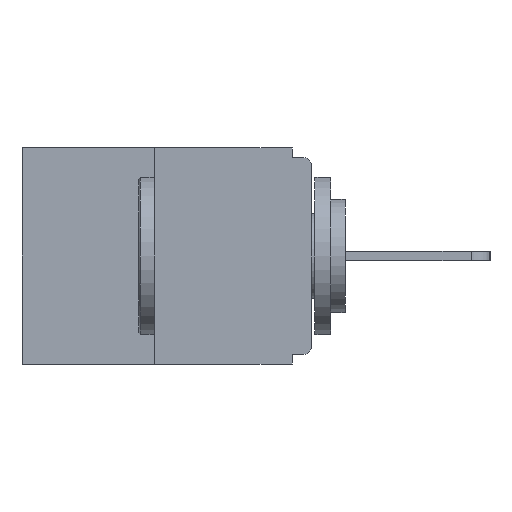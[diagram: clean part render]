
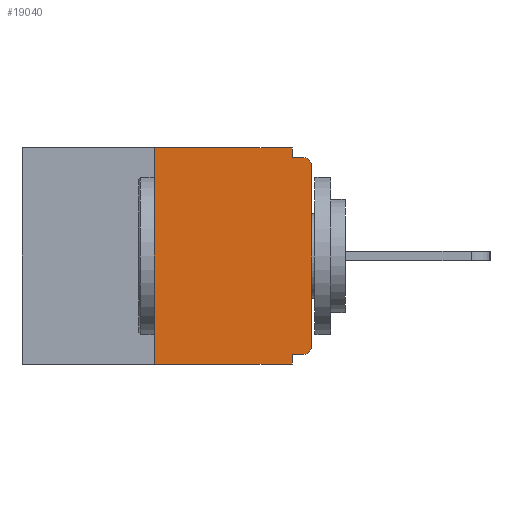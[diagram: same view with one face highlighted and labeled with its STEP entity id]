
A CAD part, left-side view. The second image highlights one B-rep face of the part: STEP entity #19040.
In plain terms, the highlighted planar face has unit normal (-1, 0, 0).
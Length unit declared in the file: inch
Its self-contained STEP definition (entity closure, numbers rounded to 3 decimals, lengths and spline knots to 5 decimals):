
#199 = VERTEX_POINT ( 'NONE', #11319 ) ;
#419 = LINE ( 'NONE', #11018, #18500 ) ;
#460 = DIRECTION ( 'NONE',  ( 1., 0., 0. ) ) ;
#535 = CARTESIAN_POINT ( 'NONE',  ( 0., 0.031, -0.343 ) ) ;
#539 = DIRECTION ( 'NONE',  ( 0., 0., -1. ) ) ;
#1986 = DIRECTION ( 'NONE',  ( 0., -1., 0. ) ) ;
#2222 = VERTEX_POINT ( 'NONE', #7398 ) ;
#2345 = CARTESIAN_POINT ( 'NONE',  ( 0., 0.46, 0. ) ) ;
#2422 = ORIENTED_EDGE ( 'NONE', *, *, #13037, .T. ) ;
#2543 = CARTESIAN_POINT ( 'NONE',  ( 0., 0., 0. ) ) ;
#2627 = VECTOR ( 'NONE', #21052, 39.37008 ) ;
#3037 = EDGE_CURVE ( 'NONE', #7523, #5427, #3733, .T. ) ;
#3152 = CARTESIAN_POINT ( 'NONE',  ( 0., 0.015, -0.03 ) ) ;
#3335 = CARTESIAN_POINT ( 'NONE',  ( 0., 0.031, -0.015 ) ) ;
#3733 = LINE ( 'NONE', #13937, #15692 ) ;
#4079 = EDGE_CURVE ( 'NONE', #18840, #16915, #9987, .T. ) ;
#4166 = ORIENTED_EDGE ( 'NONE', *, *, #6965, .F. ) ;
#4241 = DIRECTION ( 'NONE',  ( 0., -1., 0. ) ) ;
#4781 = CARTESIAN_POINT ( 'NONE',  ( 0., 0., -0.015 ) ) ;
#4887 = CARTESIAN_POINT ( 'NONE',  ( 0., 0.46, -0.343 ) ) ;
#4950 = DIRECTION ( 'NONE',  ( 0., 0., -1. ) ) ;
#5097 = DIRECTION ( 'NONE',  ( 0., 1., 0. ) ) ;
#5274 = CARTESIAN_POINT ( 'NONE',  ( 0., 0.25, 0. ) ) ;
#5427 = VERTEX_POINT ( 'NONE', #16603 ) ;
#5719 = EDGE_LOOP ( 'NONE', ( #16451, #10334, #20446, #6708, #17253, #20076, #2422, #19606, #4166, #11992 ) ) ;
#6475 = DIRECTION ( 'NONE',  ( 0., 0., 1. ) ) ;
#6708 = ORIENTED_EDGE ( 'NONE', *, *, #10070, .F. ) ;
#6965 = EDGE_CURVE ( 'NONE', #7738, #17714, #7440, .T. ) ;
#7297 = CIRCLE ( 'NONE', #14392, 0.015 ) ;
#7362 = EDGE_CURVE ( 'NONE', #199, #17811, #16793, .T. ) ;
#7398 = CARTESIAN_POINT ( 'NONE',  ( 0., 0., -0.03 ) ) ;
#7440 = LINE ( 'NONE', #4781, #19583 ) ;
#7523 = VERTEX_POINT ( 'NONE', #13383 ) ;
#7738 = VERTEX_POINT ( 'NONE', #3335 ) ;
#7961 = VECTOR ( 'NONE', #1986, 39.37008 ) ;
#8301 = EDGE_CURVE ( 'NONE', #18840, #199, #21797, .T. ) ;
#8455 = CARTESIAN_POINT ( 'NONE',  ( 0., 0., -0.313 ) ) ;
#8465 = CARTESIAN_POINT ( 'NONE',  ( 0., 0.015, -0.015 ) ) ;
#8633 = VECTOR ( 'NONE', #6475, 39.37008 ) ;
#8730 = DIRECTION ( 'NONE',  ( 0., -1., 0. ) ) ;
#8837 = EDGE_CURVE ( 'NONE', #7523, #14530, #7297, .T. ) ;
#9469 = VECTOR ( 'NONE', #8730, 39.37008 ) ;
#9909 = VECTOR ( 'NONE', #12599, 39.37008 ) ;
#9987 = LINE ( 'NONE', #4887, #9469 ) ;
#10070 = EDGE_CURVE ( 'NONE', #5427, #16915, #18637, .T. ) ;
#10184 = DIRECTION ( 'NONE',  ( 0., 0., -1. ) ) ;
#10214 = DIRECTION ( 'NONE',  ( -1., 0., 0. ) ) ;
#10334 = ORIENTED_EDGE ( 'NONE', *, *, #8301, .F. ) ;
#10362 = CARTESIAN_POINT ( 'NONE',  ( 0., 0.015, -0.313 ) ) ;
#10775 = CARTESIAN_POINT ( 'NONE',  ( 0., 0.031, 0. ) ) ;
#10934 = CARTESIAN_POINT ( 'NONE',  ( 0., 0.46, 0. ) ) ;
#11018 = CARTESIAN_POINT ( 'NONE',  ( 0., 0.031, 0. ) ) ;
#11319 = CARTESIAN_POINT ( 'NONE',  ( 0., 0.25, 0. ) ) ;
#11560 = CARTESIAN_POINT ( 'NONE',  ( 0., 0.031, -0.343 ) ) ;
#11992 = ORIENTED_EDGE ( 'NONE', *, *, #13576, .F. ) ;
#12591 = DIRECTION ( 'NONE',  ( 0., 0., -1. ) ) ;
#12599 = DIRECTION ( 'NONE',  ( 0., 0., -1. ) ) ;
#13037 = EDGE_CURVE ( 'NONE', #14530, #2222, #21090, .T. ) ;
#13159 = AXIS2_PLACEMENT_3D ( 'NONE', #10934, #460, #12591 ) ;
#13383 = CARTESIAN_POINT ( 'NONE',  ( 0., 0.015, -0.328 ) ) ;
#13576 = EDGE_CURVE ( 'NONE', #17811, #7738, #419, .T. ) ;
#13689 = CARTESIAN_POINT ( 'NONE',  ( 0., 0.25, -0.343 ) ) ;
#13937 = CARTESIAN_POINT ( 'NONE',  ( 0., 0., -0.328 ) ) ;
#14392 = AXIS2_PLACEMENT_3D ( 'NONE', #10362, #10214, #10184 ) ;
#14530 = VERTEX_POINT ( 'NONE', #8455 ) ;
#15085 = DIRECTION ( 'NONE',  ( -1., 0., 0. ) ) ;
#15692 = VECTOR ( 'NONE', #5097, 39.37008 ) ;
#16451 = ORIENTED_EDGE ( 'NONE', *, *, #7362, .F. ) ;
#16508 = EDGE_CURVE ( 'NONE', #2222, #17714, #20759, .T. ) ;
#16603 = CARTESIAN_POINT ( 'NONE',  ( 0., 0.031, -0.328 ) ) ;
#16793 = LINE ( 'NONE', #2345, #7961 ) ;
#16915 = VERTEX_POINT ( 'NONE', #11560 ) ;
#17253 = ORIENTED_EDGE ( 'NONE', *, *, #3037, .F. ) ;
#17714 = VERTEX_POINT ( 'NONE', #8465 ) ;
#17811 = VERTEX_POINT ( 'NONE', #10775 ) ;
#18500 = VECTOR ( 'NONE', #539, 39.37008 ) ;
#18637 = LINE ( 'NONE', #535, #9909 ) ;
#18840 = VERTEX_POINT ( 'NONE', #13689 ) ;
#19040 = ADVANCED_FACE ( 'NONE', ( #21168 ), #20713, .F. ) ;
#19583 = VECTOR ( 'NONE', #4241, 39.37008 ) ;
#19606 = ORIENTED_EDGE ( 'NONE', *, *, #16508, .T. ) ;
#20076 = ORIENTED_EDGE ( 'NONE', *, *, #8837, .T. ) ;
#20446 = ORIENTED_EDGE ( 'NONE', *, *, #4079, .T. ) ;
#20479 = AXIS2_PLACEMENT_3D ( 'NONE', #3152, #15085, #4950 ) ;
#20713 = PLANE ( 'NONE',  #13159 ) ;
#20759 = CIRCLE ( 'NONE', #20479, 0.015 ) ;
#21052 = DIRECTION ( 'NONE',  ( 0., 0., 1. ) ) ;
#21090 = LINE ( 'NONE', #2543, #2627 ) ;
#21168 = FACE_OUTER_BOUND ( 'NONE', #5719, .T. ) ;
#21797 = LINE ( 'NONE', #5274, #8633 ) ;
